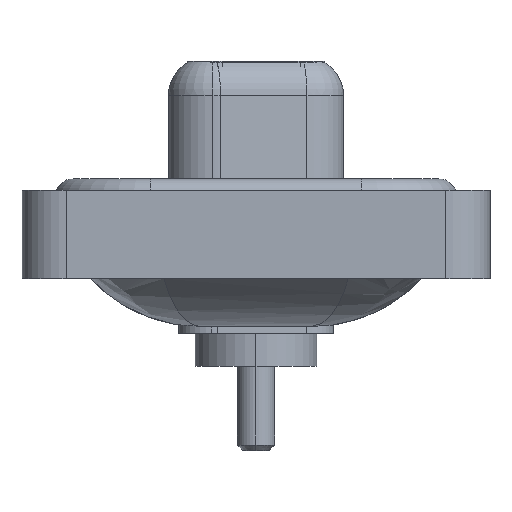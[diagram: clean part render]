
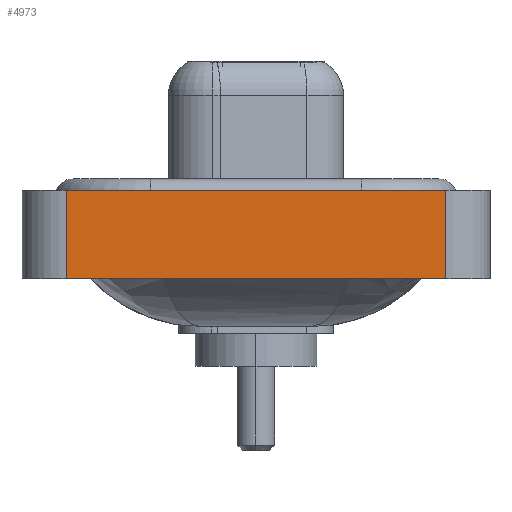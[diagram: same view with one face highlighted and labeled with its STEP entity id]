
A CAD part, left-side view. The second image highlights one B-rep face of the part: STEP entity #4973.
In plain terms, the highlighted planar face has unit normal (-1, 0, 0).
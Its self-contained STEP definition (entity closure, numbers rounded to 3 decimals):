
#496 = CARTESIAN_POINT ( 'NONE',  ( -7.35, -8.55, 0.4 ) ) ;
#751 = CARTESIAN_POINT ( 'NONE',  ( -7.35, 8.55, -3.6 ) ) ;
#1169 = ORIENTED_EDGE ( 'NONE', *, *, #7687, .F. ) ;
#2263 = VERTEX_POINT ( 'NONE', #6478 ) ;
#2733 = CARTESIAN_POINT ( 'NONE',  ( -7.35, -8.55, -3.6 ) ) ;
#2920 = CARTESIAN_POINT ( 'NONE',  ( -7.35, 8.55, 0.4 ) ) ;
#4416 = PLANE ( 'NONE',  #11613 ) ;
#4461 = EDGE_CURVE ( 'NONE', #8921, #9311, #7885, .T. ) ;
#4478 = VERTEX_POINT ( 'NONE', #496 ) ;
#4506 = EDGE_LOOP ( 'NONE', ( #6340, #1169, #10646, #16575 ) ) ;
#4615 = DIRECTION ( 'NONE',  ( 0., 0., 1. ) ) ;
#4973 = ADVANCED_FACE ( 'NONE', ( #5657 ), #4416, .T. ) ;
#5657 = FACE_OUTER_BOUND ( 'NONE', #4506, .T. ) ;
#6005 = VECTOR ( 'NONE', #9805, 1000. ) ;
#6340 = ORIENTED_EDGE ( 'NONE', *, *, #7186, .T. ) ;
#6379 = VECTOR ( 'NONE', #4615, 1000. ) ;
#6478 = CARTESIAN_POINT ( 'NONE',  ( -7.35, -8.55, -3.6 ) ) ;
#6570 = VECTOR ( 'NONE', #10373, 1000. ) ;
#7186 = EDGE_CURVE ( 'NONE', #2263, #4478, #12535, .T. ) ;
#7293 = VECTOR ( 'NONE', #12929, 1000. ) ;
#7687 = EDGE_CURVE ( 'NONE', #9311, #4478, #16449, .T. ) ;
#7885 = LINE ( 'NONE', #13267, #7293 ) ;
#8921 = VERTEX_POINT ( 'NONE', #751 ) ;
#9311 = VERTEX_POINT ( 'NONE', #2920 ) ;
#9554 = CARTESIAN_POINT ( 'NONE',  ( -7.35, -8.55, -3.6 ) ) ;
#9805 = DIRECTION ( 'NONE',  ( 0., -1., 0. ) ) ;
#10373 = DIRECTION ( 'NONE',  ( 0., -1., 0. ) ) ;
#10646 = ORIENTED_EDGE ( 'NONE', *, *, #4461, .F. ) ;
#11613 = AXIS2_PLACEMENT_3D ( 'NONE', #9554, #14677, #13416 ) ;
#11648 = LINE ( 'NONE', #2733, #6570 ) ;
#12535 = LINE ( 'NONE', #13458, #6379 ) ;
#12929 = DIRECTION ( 'NONE',  ( 0., 0., 1. ) ) ;
#13267 = CARTESIAN_POINT ( 'NONE',  ( -7.35, 8.55, -3.6 ) ) ;
#13416 = DIRECTION ( 'NONE',  ( 0., 0., 1. ) ) ;
#13458 = CARTESIAN_POINT ( 'NONE',  ( -7.35, -8.55, -3.6 ) ) ;
#13933 = CARTESIAN_POINT ( 'NONE',  ( -7.35, -8.55, 0.4 ) ) ;
#14677 = DIRECTION ( 'NONE',  ( -1., 0., 0. ) ) ;
#15453 = EDGE_CURVE ( 'NONE', #8921, #2263, #11648, .T. ) ;
#16449 = LINE ( 'NONE', #13933, #6005 ) ;
#16575 = ORIENTED_EDGE ( 'NONE', *, *, #15453, .T. ) ;
